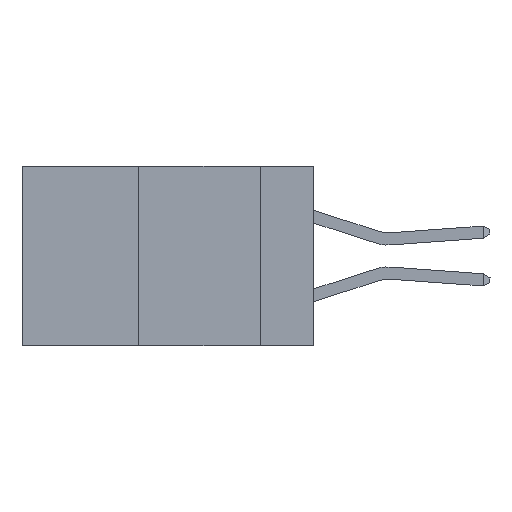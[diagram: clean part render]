
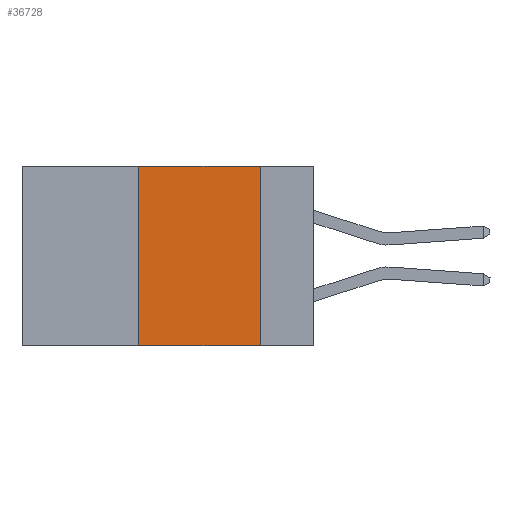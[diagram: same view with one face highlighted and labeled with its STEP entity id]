
A CAD part, left-side view. The second image highlights one B-rep face of the part: STEP entity #36728.
In plain terms, the highlighted planar face has unit normal (-1, 0, 0).
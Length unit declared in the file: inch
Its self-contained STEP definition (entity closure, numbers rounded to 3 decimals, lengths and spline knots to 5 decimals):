
#69 = LINE ( 'NONE', #11843, #35037 ) ;
#1845 = VERTEX_POINT ( 'NONE', #6880 ) ;
#1868 = CARTESIAN_POINT ( 'NONE',  ( 0., 0.11, 0. ) ) ;
#2696 = EDGE_CURVE ( 'NONE', #30377, #26785, #11046, .T. ) ;
#5600 = VECTOR ( 'NONE', #17803, 39.37008 ) ;
#6047 = DIRECTION ( 'NONE',  ( 0., 0., -1. ) ) ;
#6880 = CARTESIAN_POINT ( 'NONE',  ( 0., 0.11, -0.37 ) ) ;
#8423 = ORIENTED_EDGE ( 'NONE', *, *, #16884, .F. ) ;
#9504 = DIRECTION ( 'NONE',  ( 1., 0., 0. ) ) ;
#11046 = LINE ( 'NONE', #11995, #18385 ) ;
#11248 = AXIS2_PLACEMENT_3D ( 'NONE', #24225, #9504, #6047 ) ;
#11843 = CARTESIAN_POINT ( 'NONE',  ( 0., 0.11, 0. ) ) ;
#11995 = CARTESIAN_POINT ( 'NONE',  ( 0., 0.36, 0. ) ) ;
#12384 = PLANE ( 'NONE',  #11248 ) ;
#14266 = EDGE_CURVE ( 'NONE', #30377, #1845, #34543, .T. ) ;
#14665 = ORIENTED_EDGE ( 'NONE', *, *, #2696, .F. ) ;
#16884 = EDGE_CURVE ( 'NONE', #21060, #1845, #69, .T. ) ;
#17803 = DIRECTION ( 'NONE',  ( 0., -1., 0. ) ) ;
#18083 = ORIENTED_EDGE ( 'NONE', *, *, #14266, .T. ) ;
#18385 = VECTOR ( 'NONE', #18397, 39.37008 ) ;
#18397 = DIRECTION ( 'NONE',  ( 0., 0., 1. ) ) ;
#20358 = EDGE_CURVE ( 'NONE', #26785, #21060, #29566, .T. ) ;
#20772 = FACE_OUTER_BOUND ( 'NONE', #29359, .T. ) ;
#21060 = VERTEX_POINT ( 'NONE', #1868 ) ;
#22021 = DIRECTION ( 'NONE',  ( 0., -1., 0. ) ) ;
#23682 = DIRECTION ( 'NONE',  ( 0., 0., -1. ) ) ;
#24225 = CARTESIAN_POINT ( 'NONE',  ( 0., 0.6, 0. ) ) ;
#24962 = ORIENTED_EDGE ( 'NONE', *, *, #20358, .F. ) ;
#26173 = VECTOR ( 'NONE', #22021, 39.37008 ) ;
#26785 = VERTEX_POINT ( 'NONE', #37957 ) ;
#29359 = EDGE_LOOP ( 'NONE', ( #8423, #24962, #14665, #18083 ) ) ;
#29566 = LINE ( 'NONE', #35576, #5600 ) ;
#30377 = VERTEX_POINT ( 'NONE', #31189 ) ;
#31189 = CARTESIAN_POINT ( 'NONE',  ( 0., 0.36, -0.37 ) ) ;
#31451 = CARTESIAN_POINT ( 'NONE',  ( 0., 0.6, -0.37 ) ) ;
#34543 = LINE ( 'NONE', #31451, #26173 ) ;
#35037 = VECTOR ( 'NONE', #23682, 39.37008 ) ;
#35576 = CARTESIAN_POINT ( 'NONE',  ( 0., 0.6, 0. ) ) ;
#36728 = ADVANCED_FACE ( 'NONE', ( #20772 ), #12384, .F. ) ;
#37957 = CARTESIAN_POINT ( 'NONE',  ( 0., 0.36, 0. ) ) ;
